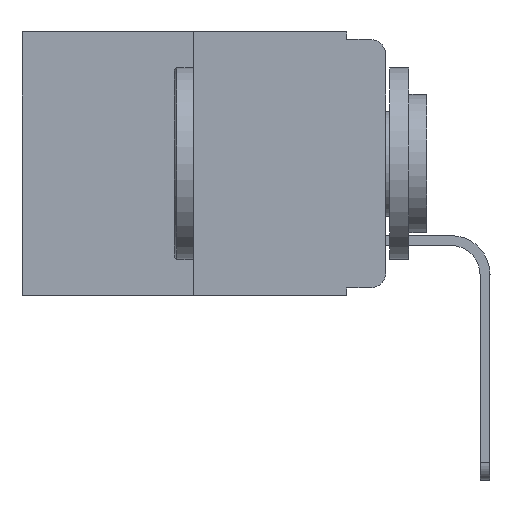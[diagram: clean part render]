
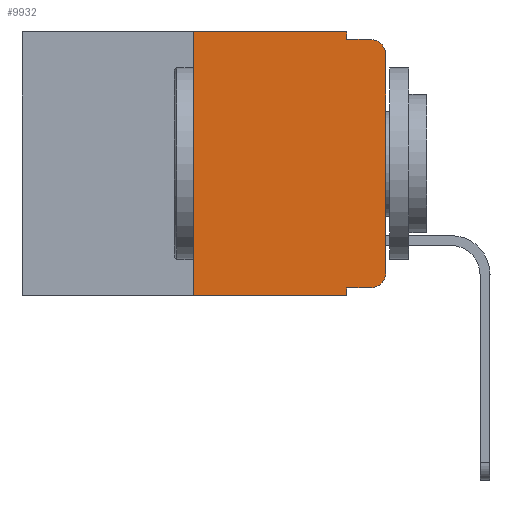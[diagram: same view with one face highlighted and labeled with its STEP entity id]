
A CAD part, left-side view. The second image highlights one B-rep face of the part: STEP entity #9932.
In plain terms, the highlighted planar face has unit normal (-1, 0, 0).
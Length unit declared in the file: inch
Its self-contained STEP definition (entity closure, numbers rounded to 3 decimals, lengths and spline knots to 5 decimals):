
#178 = VERTEX_POINT ( 'NONE', #6922 ) ;
#268 = LINE ( 'NONE', #15354, #19425 ) ;
#648 = CARTESIAN_POINT ( 'NONE',  ( 0., 0.02, -0.01 ) ) ;
#797 = LINE ( 'NONE', #9290, #16416 ) ;
#903 = EDGE_CURVE ( 'NONE', #4916, #178, #9182, .T. ) ;
#1182 = DIRECTION ( 'NONE',  ( -1., 0., 0. ) ) ;
#1737 = CARTESIAN_POINT ( 'NONE',  ( 0., 0.25, 0. ) ) ;
#1974 = CARTESIAN_POINT ( 'NONE',  ( 0., 0.051, -0.333 ) ) ;
#2040 = DIRECTION ( 'NONE',  ( 0., -1., 0. ) ) ;
#2187 = DIRECTION ( 'NONE',  ( 0., -1., 0. ) ) ;
#2216 = CARTESIAN_POINT ( 'NONE',  ( 0., 0., -0.03 ) ) ;
#2398 = VERTEX_POINT ( 'NONE', #6244 ) ;
#2962 = EDGE_LOOP ( 'NONE', ( #7337, #15999, #3307, #8402, #6346, #14132, #19288, #18829, #6289, #13109 ) ) ;
#3287 = AXIS2_PLACEMENT_3D ( 'NONE', #19376, #1182, #19435 ) ;
#3307 = ORIENTED_EDGE ( 'NONE', *, *, #7133, .F. ) ;
#3773 = FACE_OUTER_BOUND ( 'NONE', #2962, .T. ) ;
#4504 = DIRECTION ( 'NONE',  ( 0., 0., -1. ) ) ;
#4833 = VECTOR ( 'NONE', #2187, 39.37008 ) ;
#4916 = VERTEX_POINT ( 'NONE', #9811 ) ;
#5228 = CARTESIAN_POINT ( 'NONE',  ( 0., 0.051, -0.01 ) ) ;
#5241 = EDGE_CURVE ( 'NONE', #5312, #11290, #268, .T. ) ;
#5312 = VERTEX_POINT ( 'NONE', #1737 ) ;
#5556 = DIRECTION ( 'NONE',  ( 0., 0., -1. ) ) ;
#5844 = VECTOR ( 'NONE', #16032, 39.37008 ) ;
#5967 = VECTOR ( 'NONE', #2040, 39.37008 ) ;
#6109 = DIRECTION ( 'NONE',  ( 0., 0., 1. ) ) ;
#6244 = CARTESIAN_POINT ( 'NONE',  ( 0., 0.02, -0.333 ) ) ;
#6259 = EDGE_CURVE ( 'NONE', #11290, #6619, #6542, .T. ) ;
#6289 = ORIENTED_EDGE ( 'NONE', *, *, #8194, .T. ) ;
#6346 = ORIENTED_EDGE ( 'NONE', *, *, #5241, .F. ) ;
#6426 = DIRECTION ( 'NONE',  ( 1., 0., 0. ) ) ;
#6484 = AXIS2_PLACEMENT_3D ( 'NONE', #12829, #12903, #5556 ) ;
#6542 = LINE ( 'NONE', #14741, #13629 ) ;
#6619 = VERTEX_POINT ( 'NONE', #9690 ) ;
#6922 = CARTESIAN_POINT ( 'NONE',  ( 0., 0.051, -0.343 ) ) ;
#7021 = CARTESIAN_POINT ( 'NONE',  ( 0., 0., -0.313 ) ) ;
#7133 = EDGE_CURVE ( 'NONE', #6619, #8384, #13346, .T. ) ;
#7184 = DIRECTION ( 'NONE',  ( 0., 0., -1. ) ) ;
#7337 = ORIENTED_EDGE ( 'NONE', *, *, #15299, .T. ) ;
#7366 = CARTESIAN_POINT ( 'NONE',  ( 0., 0.051, 0. ) ) ;
#7606 = DIRECTION ( 'NONE',  ( 0., -1., 0. ) ) ;
#8020 = DIRECTION ( 'NONE',  ( 0., -1., 0. ) ) ;
#8194 = EDGE_CURVE ( 'NONE', #4916, #2398, #14015, .T. ) ;
#8384 = VERTEX_POINT ( 'NONE', #648 ) ;
#8402 = ORIENTED_EDGE ( 'NONE', *, *, #6259, .F. ) ;
#8587 = CIRCLE ( 'NONE', #3287, 0.02 ) ;
#9179 = VERTEX_POINT ( 'NONE', #14708 ) ;
#9182 = LINE ( 'NONE', #13173, #12246 ) ;
#9290 = CARTESIAN_POINT ( 'NONE',  ( 0., 0., 0. ) ) ;
#9350 = LINE ( 'NONE', #18925, #4833 ) ;
#9483 = CARTESIAN_POINT ( 'NONE',  ( 0., 0.473, 0. ) ) ;
#9690 = CARTESIAN_POINT ( 'NONE',  ( 0., 0.051, -0.01 ) ) ;
#9811 = CARTESIAN_POINT ( 'NONE',  ( 0., 0.051, -0.333 ) ) ;
#9932 = ADVANCED_FACE ( 'NONE', ( #3773 ), #15300, .F. ) ;
#10162 = VERTEX_POINT ( 'NONE', #2216 ) ;
#10729 = DIRECTION ( 'NONE',  ( 0., 0., -1. ) ) ;
#11290 = VERTEX_POINT ( 'NONE', #7366 ) ;
#11830 = EDGE_CURVE ( 'NONE', #9179, #5312, #13413, .T. ) ;
#11878 = VERTEX_POINT ( 'NONE', #7021 ) ;
#12246 = VECTOR ( 'NONE', #4504, 39.37008 ) ;
#12829 = CARTESIAN_POINT ( 'NONE',  ( 0., 0.02, -0.03 ) ) ;
#12903 = DIRECTION ( 'NONE',  ( -1., 0., 0. ) ) ;
#13109 = ORIENTED_EDGE ( 'NONE', *, *, #19203, .T. ) ;
#13173 = CARTESIAN_POINT ( 'NONE',  ( 0., 0.051, 0. ) ) ;
#13346 = LINE ( 'NONE', #5228, #17651 ) ;
#13375 = CIRCLE ( 'NONE', #6484, 0.02 ) ;
#13413 = LINE ( 'NONE', #14499, #5844 ) ;
#13629 = VECTOR ( 'NONE', #7184, 39.37008 ) ;
#13669 = AXIS2_PLACEMENT_3D ( 'NONE', #9483, #6426, #10729 ) ;
#13809 = EDGE_CURVE ( 'NONE', #10162, #8384, #13375, .T. ) ;
#14015 = LINE ( 'NONE', #1974, #5967 ) ;
#14132 = ORIENTED_EDGE ( 'NONE', *, *, #11830, .F. ) ;
#14322 = EDGE_CURVE ( 'NONE', #9179, #178, #9350, .T. ) ;
#14499 = CARTESIAN_POINT ( 'NONE',  ( 0., 0.25, 0. ) ) ;
#14708 = CARTESIAN_POINT ( 'NONE',  ( 0., 0.25, -0.343 ) ) ;
#14741 = CARTESIAN_POINT ( 'NONE',  ( 0., 0.051, 0. ) ) ;
#15299 = EDGE_CURVE ( 'NONE', #11878, #10162, #797, .T. ) ;
#15300 = PLANE ( 'NONE',  #13669 ) ;
#15354 = CARTESIAN_POINT ( 'NONE',  ( 0., 0.473, 0. ) ) ;
#15999 = ORIENTED_EDGE ( 'NONE', *, *, #13809, .T. ) ;
#16032 = DIRECTION ( 'NONE',  ( 0., 0., 1. ) ) ;
#16416 = VECTOR ( 'NONE', #6109, 39.37008 ) ;
#17651 = VECTOR ( 'NONE', #8020, 39.37008 ) ;
#18829 = ORIENTED_EDGE ( 'NONE', *, *, #903, .F. ) ;
#18925 = CARTESIAN_POINT ( 'NONE',  ( 0., 0.473, -0.343 ) ) ;
#19203 = EDGE_CURVE ( 'NONE', #2398, #11878, #8587, .T. ) ;
#19288 = ORIENTED_EDGE ( 'NONE', *, *, #14322, .T. ) ;
#19376 = CARTESIAN_POINT ( 'NONE',  ( 0., 0.02, -0.313 ) ) ;
#19425 = VECTOR ( 'NONE', #7606, 39.37008 ) ;
#19435 = DIRECTION ( 'NONE',  ( 0., 0., -1. ) ) ;
